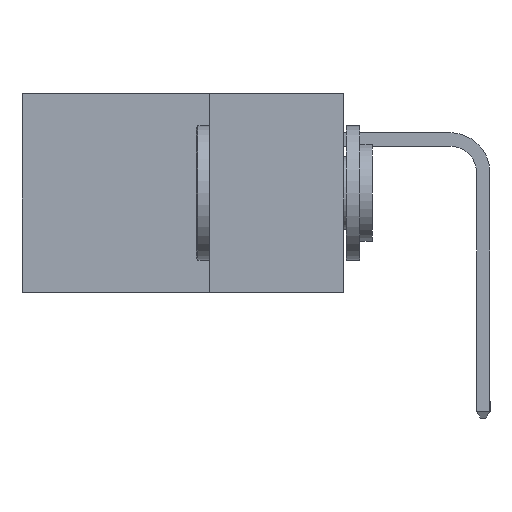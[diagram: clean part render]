
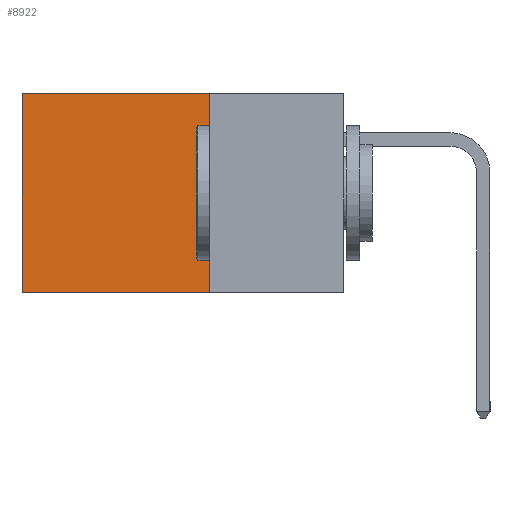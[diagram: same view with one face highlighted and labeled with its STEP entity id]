
A CAD part, left-side view. The second image highlights one B-rep face of the part: STEP entity #8922.
In plain terms, the highlighted planar face has unit normal (-1, 0, 0).
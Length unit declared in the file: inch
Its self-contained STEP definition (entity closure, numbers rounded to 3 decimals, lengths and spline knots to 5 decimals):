
#91 = FACE_OUTER_BOUND ( 'NONE', #1293, .T. ) ;
#698 = VERTEX_POINT ( 'NONE', #1565 ) ;
#1293 = EDGE_LOOP ( 'NONE', ( #4703, #6770, #2910, #1485 ) ) ;
#1465 = LINE ( 'NONE', #6913, #7450 ) ;
#1485 = ORIENTED_EDGE ( 'NONE', *, *, #7781, .T. ) ;
#1565 = CARTESIAN_POINT ( 'NONE',  ( 0.2615, 0.6, 0. ) ) ;
#1632 = LINE ( 'NONE', #1845, #7802 ) ;
#1845 = CARTESIAN_POINT ( 'NONE',  ( 0.2615, 0.25, -0.37 ) ) ;
#1948 = CARTESIAN_POINT ( 'NONE',  ( 0.2615, 0.25, -0.37 ) ) ;
#2594 = CARTESIAN_POINT ( 'NONE',  ( 0.2615, 0.25, -0.37 ) ) ;
#2699 = LINE ( 'NONE', #6649, #2948 ) ;
#2910 = ORIENTED_EDGE ( 'NONE', *, *, #4814, .F. ) ;
#2948 = VECTOR ( 'NONE', #6958, 39.37008 ) ;
#3037 = DIRECTION ( 'NONE',  ( 0., 1., 0. ) ) ;
#3104 = EDGE_CURVE ( 'NONE', #698, #7740, #2699, .T. ) ;
#3469 = DIRECTION ( 'NONE',  ( 0., 1., 0. ) ) ;
#3633 = VERTEX_POINT ( 'NONE', #1948 ) ;
#4203 = DIRECTION ( 'NONE',  ( 0., 0., -1. ) ) ;
#4703 = ORIENTED_EDGE ( 'NONE', *, *, #3104, .T. ) ;
#4814 = EDGE_CURVE ( 'NONE', #9609, #3633, #1632, .T. ) ;
#4855 = AXIS2_PLACEMENT_3D ( 'NONE', #2594, #8631, #4203 ) ;
#5399 = CARTESIAN_POINT ( 'NONE',  ( 0.2615, 0.6, -0.37 ) ) ;
#6556 = DIRECTION ( 'NONE',  ( 0., 0., -1. ) ) ;
#6643 = CARTESIAN_POINT ( 'NONE',  ( 0.2615, 0.25, 0. ) ) ;
#6649 = CARTESIAN_POINT ( 'NONE',  ( 0.2615, 0.6, -0.37 ) ) ;
#6770 = ORIENTED_EDGE ( 'NONE', *, *, #8964, .F. ) ;
#6913 = CARTESIAN_POINT ( 'NONE',  ( 0.2615, 0.25, 0. ) ) ;
#6958 = DIRECTION ( 'NONE',  ( 0., 0., -1. ) ) ;
#7450 = VECTOR ( 'NONE', #3037, 39.37008 ) ;
#7740 = VERTEX_POINT ( 'NONE', #5399 ) ;
#7759 = VECTOR ( 'NONE', #3469, 39.37008 ) ;
#7781 = EDGE_CURVE ( 'NONE', #9609, #698, #1465, .T. ) ;
#7802 = VECTOR ( 'NONE', #6556, 39.37008 ) ;
#7901 = PLANE ( 'NONE',  #4855 ) ;
#7963 = CARTESIAN_POINT ( 'NONE',  ( 0.2615, 0.25, -0.37 ) ) ;
#8631 = DIRECTION ( 'NONE',  ( 1., 0., 0. ) ) ;
#8922 = ADVANCED_FACE ( 'NONE', ( #91 ), #7901, .F. ) ;
#8964 = EDGE_CURVE ( 'NONE', #3633, #7740, #9907, .T. ) ;
#9609 = VERTEX_POINT ( 'NONE', #6643 ) ;
#9907 = LINE ( 'NONE', #7963, #7759 ) ;
